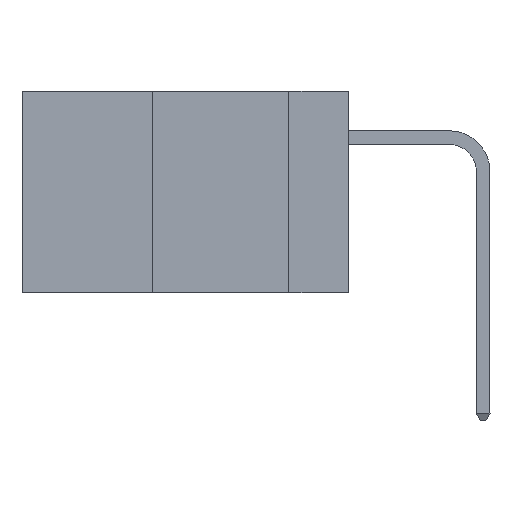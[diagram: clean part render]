
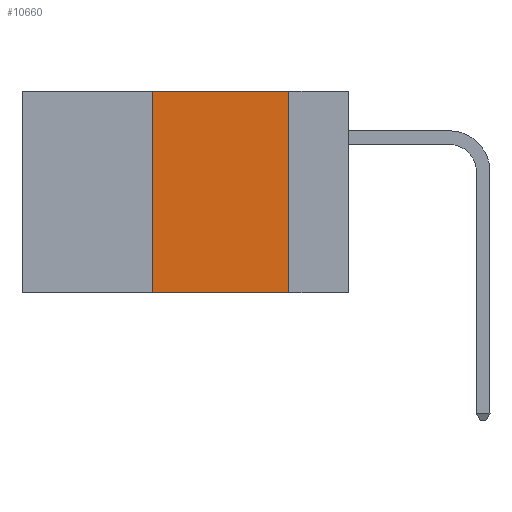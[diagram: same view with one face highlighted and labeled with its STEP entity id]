
A CAD part, left-side view. The second image highlights one B-rep face of the part: STEP entity #10660.
In plain terms, the highlighted planar face has unit normal (-1, 0, 0).
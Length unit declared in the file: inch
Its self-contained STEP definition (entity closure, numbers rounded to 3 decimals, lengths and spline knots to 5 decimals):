
#3739 = VERTEX_POINT ( 'NONE', #15149 ) ;
#3918 = CARTESIAN_POINT ( 'NONE',  ( 0., 0.11, 0. ) ) ;
#4242 = CARTESIAN_POINT ( 'NONE',  ( 0., 0.11, 0. ) ) ;
#4592 = ORIENTED_EDGE ( 'NONE', *, *, #5771, .F. ) ;
#5070 = DIRECTION ( 'NONE',  ( 1., 0., 0. ) ) ;
#5771 = EDGE_CURVE ( 'NONE', #13612, #3739, #10814, .T. ) ;
#5775 = ORIENTED_EDGE ( 'NONE', *, *, #20650, .F. ) ;
#6153 = EDGE_CURVE ( 'NONE', #17997, #3739, #20954, .T. ) ;
#7217 = LINE ( 'NONE', #19436, #19442 ) ;
#7298 = DIRECTION ( 'NONE',  ( 0., 0., -1. ) ) ;
#8917 = DIRECTION ( 'NONE',  ( 0., 0., 1. ) ) ;
#10660 = ADVANCED_FACE ( 'NONE', ( #15048 ), #13689, .F. ) ;
#10814 = LINE ( 'NONE', #4242, #22253 ) ;
#11000 = CARTESIAN_POINT ( 'NONE',  ( 0., 0.6, -0.37 ) ) ;
#11466 = DIRECTION ( 'NONE',  ( 0., -1., 0. ) ) ;
#11560 = VECTOR ( 'NONE', #11466, 39.37008 ) ;
#12963 = CARTESIAN_POINT ( 'NONE',  ( 0., 0.36, -0.37 ) ) ;
#13612 = VERTEX_POINT ( 'NONE', #3918 ) ;
#13689 = PLANE ( 'NONE',  #21439 ) ;
#14536 = VERTEX_POINT ( 'NONE', #20824 ) ;
#15048 = FACE_OUTER_BOUND ( 'NONE', #18375, .T. ) ;
#15149 = CARTESIAN_POINT ( 'NONE',  ( 0., 0.11, -0.37 ) ) ;
#15689 = ORIENTED_EDGE ( 'NONE', *, *, #6153, .T. ) ;
#17389 = EDGE_CURVE ( 'NONE', #17997, #14536, #7217, .T. ) ;
#17926 = VECTOR ( 'NONE', #21179, 39.37008 ) ;
#17997 = VERTEX_POINT ( 'NONE', #12963 ) ;
#18338 = ORIENTED_EDGE ( 'NONE', *, *, #17389, .F. ) ;
#18375 = EDGE_LOOP ( 'NONE', ( #4592, #5775, #18338, #15689 ) ) ;
#18700 = CARTESIAN_POINT ( 'NONE',  ( 0., 0.6, 0. ) ) ;
#18870 = DIRECTION ( 'NONE',  ( 0., 0., -1. ) ) ;
#19436 = CARTESIAN_POINT ( 'NONE',  ( 0., 0.36, 0. ) ) ;
#19442 = VECTOR ( 'NONE', #8917, 39.37008 ) ;
#20573 = CARTESIAN_POINT ( 'NONE',  ( 0., 0.6, 0. ) ) ;
#20650 = EDGE_CURVE ( 'NONE', #14536, #13612, #21979, .T. ) ;
#20824 = CARTESIAN_POINT ( 'NONE',  ( 0., 0.36, 0. ) ) ;
#20954 = LINE ( 'NONE', #11000, #17926 ) ;
#21179 = DIRECTION ( 'NONE',  ( 0., -1., 0. ) ) ;
#21439 = AXIS2_PLACEMENT_3D ( 'NONE', #20573, #5070, #18870 ) ;
#21979 = LINE ( 'NONE', #18700, #11560 ) ;
#22253 = VECTOR ( 'NONE', #7298, 39.37008 ) ;
